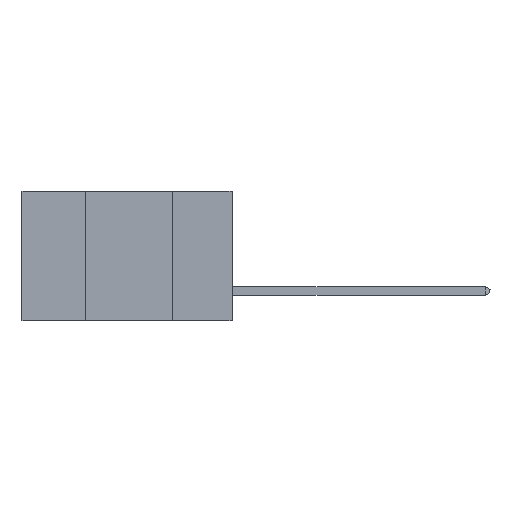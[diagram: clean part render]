
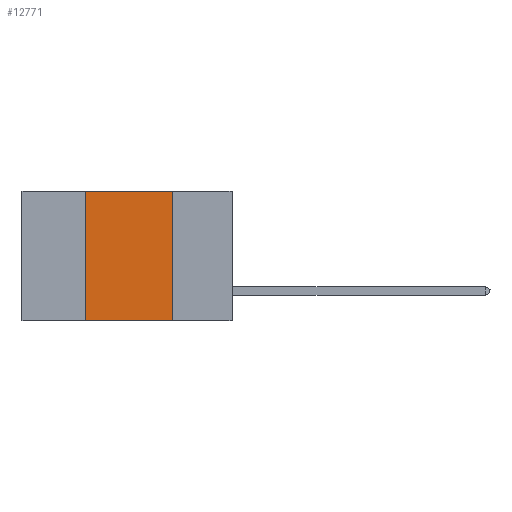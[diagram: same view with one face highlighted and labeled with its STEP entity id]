
A CAD part, left-side view. The second image highlights one B-rep face of the part: STEP entity #12771.
In plain terms, the highlighted planar face has unit normal (-1, 0, 0).
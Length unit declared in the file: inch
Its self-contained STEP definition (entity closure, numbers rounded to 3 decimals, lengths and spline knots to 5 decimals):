
#324 = DIRECTION ( 'NONE',  ( 0., -1., 0. ) ) ;
#1478 = AXIS2_PLACEMENT_3D ( 'NONE', #9727, #9531, #17569 ) ;
#1785 = CARTESIAN_POINT ( 'NONE',  ( 0., 0.42, -0.37 ) ) ;
#1944 = CARTESIAN_POINT ( 'NONE',  ( 0., 0.6, -0.37 ) ) ;
#2988 = LINE ( 'NONE', #15440, #9538 ) ;
#4226 = FACE_OUTER_BOUND ( 'NONE', #4914, .T. ) ;
#4693 = CARTESIAN_POINT ( 'NONE',  ( 0., 0.17, 0. ) ) ;
#4796 = ORIENTED_EDGE ( 'NONE', *, *, #12997, .F. ) ;
#4914 = EDGE_LOOP ( 'NONE', ( #5663, #19173, #4796, #11405 ) ) ;
#5199 = CARTESIAN_POINT ( 'NONE',  ( 0., 0.17, -0.37 ) ) ;
#5663 = ORIENTED_EDGE ( 'NONE', *, *, #12166, .F. ) ;
#6229 = CARTESIAN_POINT ( 'NONE',  ( 0., 0.42, 0. ) ) ;
#6809 = LINE ( 'NONE', #6229, #14805 ) ;
#7755 = EDGE_CURVE ( 'NONE', #14754, #19904, #8404, .T. ) ;
#8392 = VERTEX_POINT ( 'NONE', #10394 ) ;
#8404 = LINE ( 'NONE', #1944, #19016 ) ;
#9104 = EDGE_CURVE ( 'NONE', #8392, #9860, #2988, .T. ) ;
#9246 = DIRECTION ( 'NONE',  ( 0., 0., -1. ) ) ;
#9531 = DIRECTION ( 'NONE',  ( 1., 0., 0. ) ) ;
#9538 = VECTOR ( 'NONE', #324, 39.37008 ) ;
#9727 = CARTESIAN_POINT ( 'NONE',  ( 0., 0.6, 0. ) ) ;
#9860 = VERTEX_POINT ( 'NONE', #4693 ) ;
#10394 = CARTESIAN_POINT ( 'NONE',  ( 0., 0.42, 0. ) ) ;
#11405 = ORIENTED_EDGE ( 'NONE', *, *, #7755, .T. ) ;
#11560 = VECTOR ( 'NONE', #9246, 39.37008 ) ;
#12166 = EDGE_CURVE ( 'NONE', #9860, #19904, #17382, .T. ) ;
#12462 = DIRECTION ( 'NONE',  ( 0., 0., 1. ) ) ;
#12536 = DIRECTION ( 'NONE',  ( 0., -1., 0. ) ) ;
#12711 = PLANE ( 'NONE',  #1478 ) ;
#12771 = ADVANCED_FACE ( 'NONE', ( #4226 ), #12711, .F. ) ;
#12997 = EDGE_CURVE ( 'NONE', #14754, #8392, #6809, .T. ) ;
#14754 = VERTEX_POINT ( 'NONE', #1785 ) ;
#14805 = VECTOR ( 'NONE', #12462, 39.37008 ) ;
#15440 = CARTESIAN_POINT ( 'NONE',  ( 0., 0.6, 0. ) ) ;
#17382 = LINE ( 'NONE', #18474, #11560 ) ;
#17569 = DIRECTION ( 'NONE',  ( 0., 0., -1. ) ) ;
#18474 = CARTESIAN_POINT ( 'NONE',  ( 0., 0.17, 0. ) ) ;
#19016 = VECTOR ( 'NONE', #12536, 39.37008 ) ;
#19173 = ORIENTED_EDGE ( 'NONE', *, *, #9104, .F. ) ;
#19904 = VERTEX_POINT ( 'NONE', #5199 ) ;
